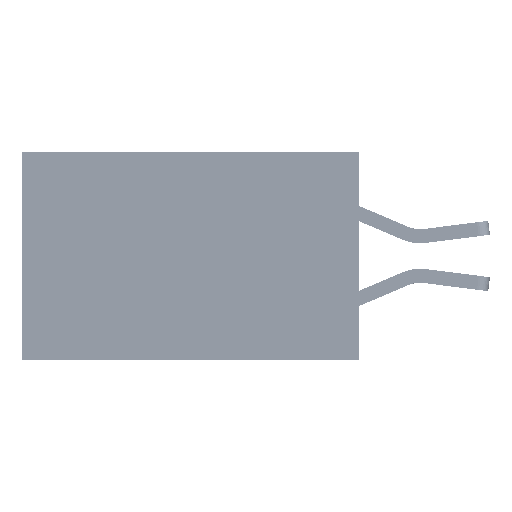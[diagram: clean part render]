
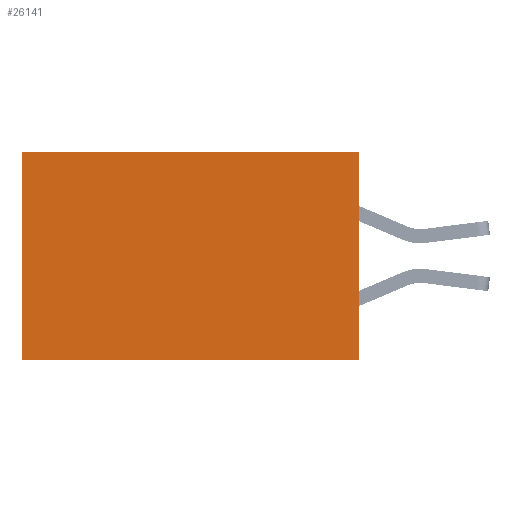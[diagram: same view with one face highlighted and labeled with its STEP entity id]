
A CAD part, left-side view. The second image highlights one B-rep face of the part: STEP entity #26141.
In plain terms, the highlighted planar face has unit normal (-1, 0, 0).
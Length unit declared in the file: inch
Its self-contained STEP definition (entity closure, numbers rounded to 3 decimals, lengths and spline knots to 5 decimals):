
#53 = VERTEX_POINT ( 'NONE', #35188 ) ;
#614 = ORIENTED_EDGE ( 'NONE', *, *, #10543, .T. ) ;
#1097 = EDGE_CURVE ( 'NONE', #6421, #53, #13427, .T. ) ;
#2375 = FACE_OUTER_BOUND ( 'NONE', #25644, .T. ) ;
#2454 = VERTEX_POINT ( 'NONE', #39027 ) ;
#3703 = EDGE_CURVE ( 'NONE', #53, #17783, #16135, .T. ) ;
#3919 = VECTOR ( 'NONE', #15765, 39.37008 ) ;
#6421 = VERTEX_POINT ( 'NONE', #13587 ) ;
#6666 = CARTESIAN_POINT ( 'NONE',  ( 0.2875, 0.6, -0.37 ) ) ;
#6840 = ORIENTED_EDGE ( 'NONE', *, *, #23298, .T. ) ;
#10543 = EDGE_CURVE ( 'NONE', #6421, #2454, #12193, .T. ) ;
#12193 = LINE ( 'NONE', #28112, #3919 ) ;
#13427 = LINE ( 'NONE', #40136, #20721 ) ;
#13587 = CARTESIAN_POINT ( 'NONE',  ( 0.2875, 0., 0. ) ) ;
#15308 = DIRECTION ( 'NONE',  ( 0., 0., -1. ) ) ;
#15765 = DIRECTION ( 'NONE',  ( 0., 1., 0. ) ) ;
#16003 = CARTESIAN_POINT ( 'NONE',  ( 0.2875, 0., 0. ) ) ;
#16135 = LINE ( 'NONE', #29603, #39920 ) ;
#17436 = ORIENTED_EDGE ( 'NONE', *, *, #3703, .F. ) ;
#17542 = DIRECTION ( 'NONE',  ( 0., 0., -1. ) ) ;
#17783 = VERTEX_POINT ( 'NONE', #6666 ) ;
#18627 = LINE ( 'NONE', #33000, #33183 ) ;
#19122 = DIRECTION ( 'NONE',  ( 0., 0., -1. ) ) ;
#20274 = ORIENTED_EDGE ( 'NONE', *, *, #1097, .F. ) ;
#20721 = VECTOR ( 'NONE', #15308, 39.37008 ) ;
#23298 = EDGE_CURVE ( 'NONE', #2454, #17783, #18627, .T. ) ;
#25644 = EDGE_LOOP ( 'NONE', ( #6840, #17436, #20274, #614 ) ) ;
#26141 = ADVANCED_FACE ( 'NONE', ( #2375 ), #34589, .F. ) ;
#28112 = CARTESIAN_POINT ( 'NONE',  ( 0.2875, 0., 0. ) ) ;
#29603 = CARTESIAN_POINT ( 'NONE',  ( 0.2875, 0., -0.37 ) ) ;
#31133 = AXIS2_PLACEMENT_3D ( 'NONE', #16003, #37702, #19122 ) ;
#32715 = DIRECTION ( 'NONE',  ( 0., 1., 0. ) ) ;
#33000 = CARTESIAN_POINT ( 'NONE',  ( 0.2875, 0.6, 0. ) ) ;
#33183 = VECTOR ( 'NONE', #17542, 39.37008 ) ;
#34589 = PLANE ( 'NONE',  #31133 ) ;
#35188 = CARTESIAN_POINT ( 'NONE',  ( 0.2875, 0., -0.37 ) ) ;
#37702 = DIRECTION ( 'NONE',  ( 1., 0., 0. ) ) ;
#39027 = CARTESIAN_POINT ( 'NONE',  ( 0.2875, 0.6, 0. ) ) ;
#39920 = VECTOR ( 'NONE', #32715, 39.37008 ) ;
#40136 = CARTESIAN_POINT ( 'NONE',  ( 0.2875, 0., 0. ) ) ;
